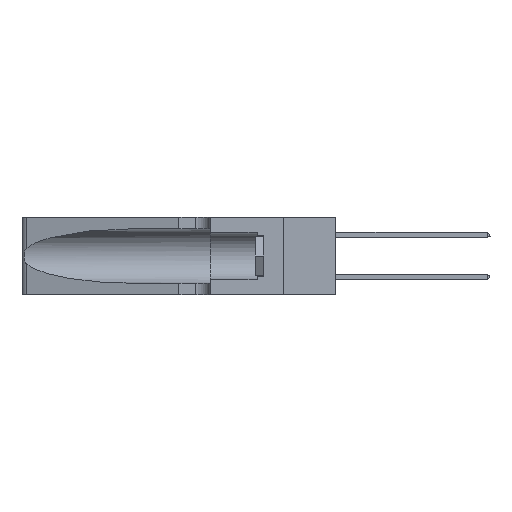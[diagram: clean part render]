
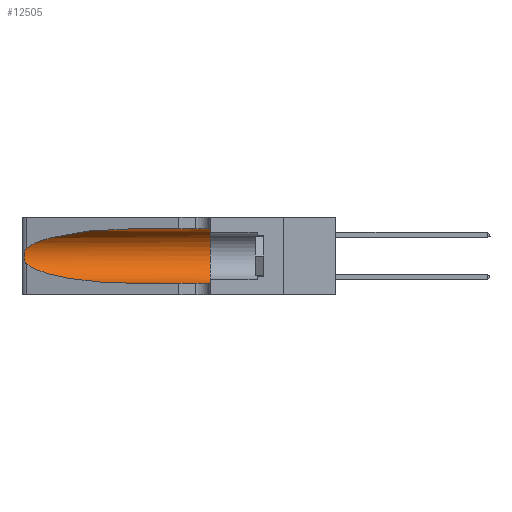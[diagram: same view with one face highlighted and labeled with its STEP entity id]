
A CAD part, left-side view. The second image highlights one B-rep face of the part: STEP entity #12505.
In plain terms, the highlighted cylindrical face has radius 3.308 mm (diameter 6.617 mm), a partial arc.
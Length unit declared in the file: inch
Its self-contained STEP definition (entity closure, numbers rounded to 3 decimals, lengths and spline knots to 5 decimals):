
#566 = DIRECTION ( 'NONE',  ( 0., 1., 0. ) ) ;
#1381 = CARTESIAN_POINT ( 'NONE',  ( 0.2373, 1.15595, 0.08982 ) ) ;
#1986 = ORIENTED_EDGE ( 'NONE', *, *, #9465, .T. ) ;
#2268 = CARTESIAN_POINT ( 'NONE',  ( 0.25787, 1.23484, 0.2124 ) ) ;
#2388 = DIRECTION ( 'NONE',  ( 0., 0., -1. ) ) ;
#2536 = ORIENTED_EDGE ( 'NONE', *, *, #27014, .F. ) ;
#2585 = ORIENTED_EDGE ( 'NONE', *, *, #11640, .T. ) ;
#2718 = VERTEX_POINT ( 'NONE', #18382 ) ;
#3116 = VERTEX_POINT ( 'NONE', #23780 ) ;
#3178 = EDGE_CURVE ( 'NONE', #3116, #7647, #14473, .T. ) ;
#4517 = CARTESIAN_POINT ( 'NONE',  ( 0.26018, 1.23835, 0.19895 ) ) ;
#5013 = CYLINDRICAL_SURFACE ( 'NONE', #9686, 0.13025 ) ;
#5908 = CARTESIAN_POINT ( 'NONE',  ( 0.1305, 0.72297, 0.05475 ) ) ;
#6763 = CARTESIAN_POINT ( 'NONE',  ( 0.26075, 1.23896, 0.178 ) ) ;
#6949 = CARTESIAN_POINT ( 'NONE',  ( 0.1305, 0.35, 0.05475 ) ) ;
#7647 = VERTEX_POINT ( 'NONE', #22664 ) ;
#8062 = CARTESIAN_POINT ( 'NONE',  ( 0.25487, 1.22718, 0.14631 ) ) ;
#8589 = CARTESIAN_POINT ( 'NONE',  ( 0.25487, 1.22718, 0.22369 ) ) ;
#8822 = EDGE_CURVE ( 'NONE', #15473, #11291, #26575, .T. ) ;
#8996 = CARTESIAN_POINT ( 'NONE',  ( 0.25856, 1.23593, 0.16098 ) ) ;
#9465 = EDGE_CURVE ( 'NONE', #7647, #15473, #22458, .T. ) ;
#9686 = AXIS2_PLACEMENT_3D ( 'NONE', #19922, #15645, #2388 ) ;
#10131 = ORIENTED_EDGE ( 'NONE', *, *, #8822, .T. ) ;
#10361 = CARTESIAN_POINT ( 'NONE',  ( 0.1305, 1.61858, 0.05475 ) ) ;
#10485 = LINE ( 'NONE', #19058, #21355 ) ;
#10846 = AXIS2_PLACEMENT_3D ( 'NONE', #13933, #566, #16093 ) ;
#11141 = CARTESIAN_POINT ( 'NONE',  ( 0.25555, 1.22994, 0.2215 ) ) ;
#11237 = CARTESIAN_POINT ( 'NONE',  ( 0.25639, 1.23186, 0.15144 ) ) ;
#11291 = VERTEX_POINT ( 'NONE', #6949 ) ;
#11640 = EDGE_CURVE ( 'NONE', #2718, #3116, #12379, .T. ) ;
#12236 = ORIENTED_EDGE ( 'NONE', *, *, #3178, .T. ) ;
#12379 =( BOUNDED_CURVE ( )  B_SPLINE_CURVE ( 3, ( #25914, #19493, #21662, #8589 ),
 .UNSPECIFIED., .F., .T. ) 
 B_SPLINE_CURVE_WITH_KNOTS ( ( 4, 4 ),
 ( 1.5708, 2.84003 ),
 .UNSPECIFIED. ) 
 CURVE ( )  GEOMETRIC_REPRESENTATION_ITEM ( )  RATIONAL_B_SPLINE_CURVE ( ( 1., 0.87, 0.87, 1. ) ) 
 REPRESENTATION_ITEM ( '' )  );
#12505 = ADVANCED_FACE ( 'NONE', ( #22493 ), #5013, .F. ) ;
#12938 = CIRCLE ( 'NONE', #10846, 0.13025 ) ;
#13186 = CARTESIAN_POINT ( 'NONE',  ( 0.1305, 0.72297, 0.05475 ) ) ;
#13452 = CARTESIAN_POINT ( 'NONE',  ( 0.25487, 1.22718, 0.14631 ) ) ;
#13933 = CARTESIAN_POINT ( 'NONE',  ( 0.1305, 0.35, 0.185 ) ) ;
#14473 = B_SPLINE_CURVE_WITH_KNOTS ( 'NONE', 3,
 ( #26307, #11141, #15518, #2268, #17698, #4517, #19884, #6763, #22052, #8996, #24244, #11237, #26398, #13452 ),
 .UNSPECIFIED., .F., .F.,
 ( 4, 2, 2, 2, 2, 2, 4 ),
 ( 0., 0.00027, 0.00053, 0.00107, 0.0016, 0.00187, 0.00214 ),
 .UNSPECIFIED. ) ;
#15415 = EDGE_LOOP ( 'NONE', ( #2585, #12236, #1986, #10131, #21617, #2536 ) ) ;
#15473 = VERTEX_POINT ( 'NONE', #13186 ) ;
#15518 = CARTESIAN_POINT ( 'NONE',  ( 0.25639, 1.23184, 0.21858 ) ) ;
#15645 = DIRECTION ( 'NONE',  ( 0., -1., 0. ) ) ;
#16093 = DIRECTION ( 'NONE',  ( 0., 0., 1. ) ) ;
#17698 = CARTESIAN_POINT ( 'NONE',  ( 0.25854, 1.2359, 0.20912 ) ) ;
#18382 = CARTESIAN_POINT ( 'NONE',  ( 0.1305, 0.72297, 0.31525 ) ) ;
#19008 = DIRECTION ( 'NONE',  ( 0., -1., 0. ) ) ;
#19058 = CARTESIAN_POINT ( 'NONE',  ( 0.1305, 1.61858, 0.31525 ) ) ;
#19066 = CARTESIAN_POINT ( 'NONE',  ( 0.18966, 0.96281, 0.05475 ) ) ;
#19493 = CARTESIAN_POINT ( 'NONE',  ( 0.18966, 0.96281, 0.31525 ) ) ;
#19884 = CARTESIAN_POINT ( 'NONE',  ( 0.26075, 1.23896, 0.19203 ) ) ;
#19922 = CARTESIAN_POINT ( 'NONE',  ( 0.1305, 1.61858, 0.185 ) ) ;
#21221 = DIRECTION ( 'NONE',  ( 0., -1., 0. ) ) ;
#21355 = VECTOR ( 'NONE', #21221, 39.37008 ) ;
#21617 = ORIENTED_EDGE ( 'NONE', *, *, #25631, .F. ) ;
#21662 = CARTESIAN_POINT ( 'NONE',  ( 0.2373, 1.15595, 0.28018 ) ) ;
#22052 = CARTESIAN_POINT ( 'NONE',  ( 0.26017, 1.23833, 0.17102 ) ) ;
#22458 =( BOUNDED_CURVE ( )  B_SPLINE_CURVE ( 3, ( #8062, #1381, #19066, #5908 ),
 .UNSPECIFIED., .F., .F. ) 
 B_SPLINE_CURVE_WITH_KNOTS ( ( 4, 4 ),
 ( 3.44316, 4.71239 ),
 .UNSPECIFIED. ) 
 CURVE ( )  GEOMETRIC_REPRESENTATION_ITEM ( )  RATIONAL_B_SPLINE_CURVE ( ( 1., 0.87, 0.87, 1. ) ) 
 REPRESENTATION_ITEM ( '' )  );
#22493 = FACE_OUTER_BOUND ( 'NONE', #15415, .T. ) ;
#22664 = CARTESIAN_POINT ( 'NONE',  ( 0.25487, 1.22718, 0.14631 ) ) ;
#23780 = CARTESIAN_POINT ( 'NONE',  ( 0.25487, 1.22718, 0.22369 ) ) ;
#24244 = CARTESIAN_POINT ( 'NONE',  ( 0.25789, 1.23486, 0.15765 ) ) ;
#25265 = VERTEX_POINT ( 'NONE', #27858 ) ;
#25631 = EDGE_CURVE ( 'NONE', #25265, #11291, #12938, .T. ) ;
#25908 = VECTOR ( 'NONE', #19008, 39.37008 ) ;
#25914 = CARTESIAN_POINT ( 'NONE',  ( 0.1305, 0.72297, 0.31525 ) ) ;
#26307 = CARTESIAN_POINT ( 'NONE',  ( 0.25487, 1.22718, 0.22369 ) ) ;
#26398 = CARTESIAN_POINT ( 'NONE',  ( 0.25555, 1.22993, 0.14849 ) ) ;
#26575 = LINE ( 'NONE', #10361, #25908 ) ;
#27014 = EDGE_CURVE ( 'NONE', #2718, #25265, #10485, .T. ) ;
#27858 = CARTESIAN_POINT ( 'NONE',  ( 0.1305, 0.35, 0.31525 ) ) ;
